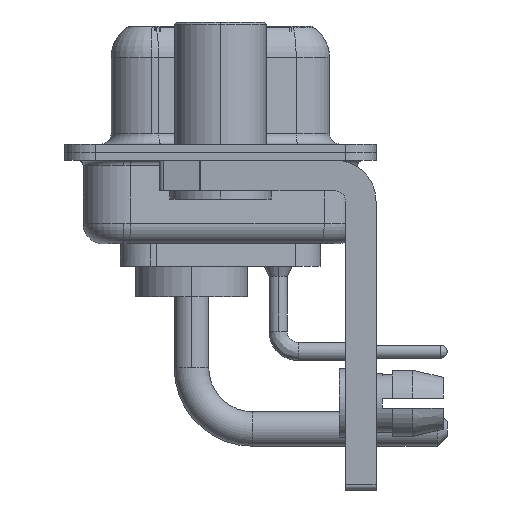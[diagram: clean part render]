
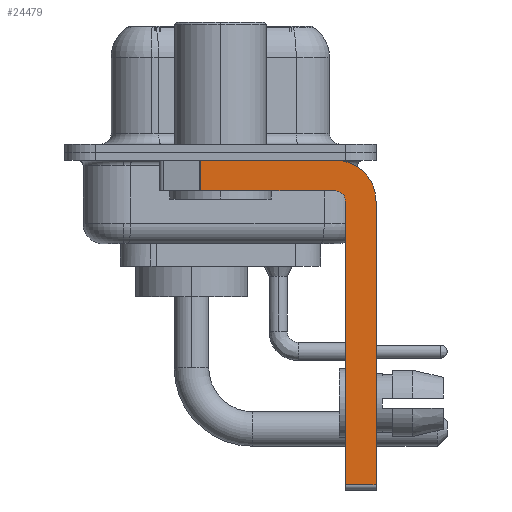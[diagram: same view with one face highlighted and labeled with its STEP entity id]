
A CAD part, left-side view. The second image highlights one B-rep face of the part: STEP entity #24479.
In plain terms, the highlighted planar face has unit normal (-1, 0, 0).
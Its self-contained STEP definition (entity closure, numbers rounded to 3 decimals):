
#476 = VERTEX_POINT ( 'NONE', #13827 ) ;
#513 = VECTOR ( 'NONE', #14098, 1000. ) ;
#1254 = EDGE_CURVE ( 'NONE', #7613, #24700, #1774, .T. ) ;
#1774 = CIRCLE ( 'NONE', #3358, 0.5 ) ;
#2107 = ORIENTED_EDGE ( 'NONE', *, *, #18172, .F. ) ;
#2208 = CARTESIAN_POINT ( 'NONE',  ( -2.9, -5.65, -1.9 ) ) ;
#2665 = ORIENTED_EDGE ( 'NONE', *, *, #16377, .T. ) ;
#2797 = LINE ( 'NONE', #10312, #19499 ) ;
#3223 = ORIENTED_EDGE ( 'NONE', *, *, #14832, .F. ) ;
#3294 = DIRECTION ( 'NONE',  ( 0., -1., 0. ) ) ;
#3358 = AXIS2_PLACEMENT_3D ( 'NONE', #22918, #18664, #9120 ) ;
#3515 = LINE ( 'NONE', #11148, #17624 ) ;
#3638 = DIRECTION ( 'NONE',  ( 0., 0., -1. ) ) ;
#5506 = VERTEX_POINT ( 'NONE', #17207 ) ;
#6608 = LINE ( 'NONE', #19451, #513 ) ;
#6872 = CARTESIAN_POINT ( 'NONE',  ( -2.9, -7.65, -2.4 ) ) ;
#7055 = LINE ( 'NONE', #14671, #24240 ) ;
#7613 = VERTEX_POINT ( 'NONE', #14515 ) ;
#7740 = ORIENTED_EDGE ( 'NONE', *, *, #12925, .T. ) ;
#8188 = AXIS2_PLACEMENT_3D ( 'NONE', #19850, #8419, #12545 ) ;
#8419 = DIRECTION ( 'NONE',  ( 1., 0., 0. ) ) ;
#9088 = CARTESIAN_POINT ( 'NONE',  ( -2.9, -5.65, -1.9 ) ) ;
#9120 = DIRECTION ( 'NONE',  ( 0., 0., 1. ) ) ;
#9176 = EDGE_CURVE ( 'NONE', #10939, #476, #3515, .T. ) ;
#9474 = DIRECTION ( 'NONE',  ( 1., 0., 0. ) ) ;
#9880 = AXIS2_PLACEMENT_3D ( 'NONE', #20877, #9474, #13338 ) ;
#10312 = CARTESIAN_POINT ( 'NONE',  ( -2.9, -6.15, -16.6 ) ) ;
#10663 = ORIENTED_EDGE ( 'NONE', *, *, #14984, .F. ) ;
#10939 = VERTEX_POINT ( 'NONE', #6872 ) ;
#10964 = LINE ( 'NONE', #9088, #17339 ) ;
#11148 = CARTESIAN_POINT ( 'NONE',  ( -2.9, -7.65, -2.4 ) ) ;
#11369 = CIRCLE ( 'NONE', #8188, 2. ) ;
#11480 = CARTESIAN_POINT ( 'NONE',  ( -2.9, -5.65, -0.4 ) ) ;
#12545 = DIRECTION ( 'NONE',  ( 0., 0., -1. ) ) ;
#12914 = VERTEX_POINT ( 'NONE', #20571 ) ;
#12925 = EDGE_CURVE ( 'NONE', #5506, #22985, #6608, .T. ) ;
#13221 = ORIENTED_EDGE ( 'NONE', *, *, #9176, .F. ) ;
#13338 = DIRECTION ( 'NONE',  ( 0., 0., -1. ) ) ;
#13683 = DIRECTION ( 'NONE',  ( 0., -1., 0. ) ) ;
#13827 = CARTESIAN_POINT ( 'NONE',  ( -2.9, -7.65, -16.35 ) ) ;
#14098 = DIRECTION ( 'NONE',  ( 0., 0., -1. ) ) ;
#14515 = CARTESIAN_POINT ( 'NONE',  ( -2.9, -6.15, -2.4 ) ) ;
#14671 = CARTESIAN_POINT ( 'NONE',  ( -2.9, -5.65, -16.35 ) ) ;
#14832 = EDGE_CURVE ( 'NONE', #5506, #18803, #15823, .T. ) ;
#14984 = EDGE_CURVE ( 'NONE', #18803, #10939, #11369, .T. ) ;
#15823 = LINE ( 'NONE', #17602, #21788 ) ;
#16377 = EDGE_CURVE ( 'NONE', #12914, #476, #7055, .T. ) ;
#16489 = CARTESIAN_POINT ( 'NONE',  ( -2.9, 0.978, -1.9 ) ) ;
#17207 = CARTESIAN_POINT ( 'NONE',  ( -2.9, 0.978, -0.4 ) ) ;
#17339 = VECTOR ( 'NONE', #18632, 1000. ) ;
#17602 = CARTESIAN_POINT ( 'NONE',  ( -2.9, 3., -0.4 ) ) ;
#17624 = VECTOR ( 'NONE', #3638, 1000. ) ;
#18172 = EDGE_CURVE ( 'NONE', #12914, #7613, #2797, .T. ) ;
#18217 = DIRECTION ( 'NONE',  ( 0., 0., 1. ) ) ;
#18514 = FACE_OUTER_BOUND ( 'NONE', #23993, .T. ) ;
#18632 = DIRECTION ( 'NONE',  ( 0., 1., 0. ) ) ;
#18664 = DIRECTION ( 'NONE',  ( -1., 0., 0. ) ) ;
#18803 = VERTEX_POINT ( 'NONE', #11480 ) ;
#19451 = CARTESIAN_POINT ( 'NONE',  ( -2.9, 0.978, -1.9 ) ) ;
#19499 = VECTOR ( 'NONE', #18217, 1000. ) ;
#19850 = CARTESIAN_POINT ( 'NONE',  ( -2.9, -5.65, -2.4 ) ) ;
#20145 = ORIENTED_EDGE ( 'NONE', *, *, #20527, .F. ) ;
#20527 = EDGE_CURVE ( 'NONE', #24700, #22985, #10964, .T. ) ;
#20571 = CARTESIAN_POINT ( 'NONE',  ( -2.9, -6.15, -16.35 ) ) ;
#20633 = PLANE ( 'NONE',  #9880 ) ;
#20877 = CARTESIAN_POINT ( 'NONE',  ( -2.9, -5.65, -2.4 ) ) ;
#21788 = VECTOR ( 'NONE', #13683, 1000. ) ;
#22918 = CARTESIAN_POINT ( 'NONE',  ( -2.9, -5.65, -2.4 ) ) ;
#22985 = VERTEX_POINT ( 'NONE', #16489 ) ;
#23993 = EDGE_LOOP ( 'NONE', ( #3223, #7740, #20145, #24298, #2107, #2665, #13221, #10663 ) ) ;
#24240 = VECTOR ( 'NONE', #3294, 1000. ) ;
#24298 = ORIENTED_EDGE ( 'NONE', *, *, #1254, .F. ) ;
#24479 = ADVANCED_FACE ( 'NONE', ( #18514 ), #20633, .F. ) ;
#24700 = VERTEX_POINT ( 'NONE', #2208 ) ;
